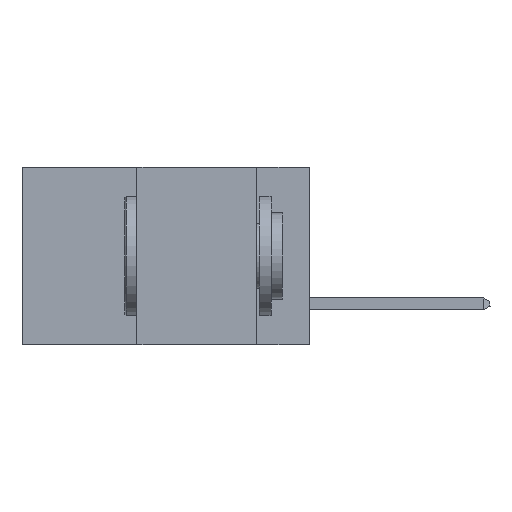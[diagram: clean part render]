
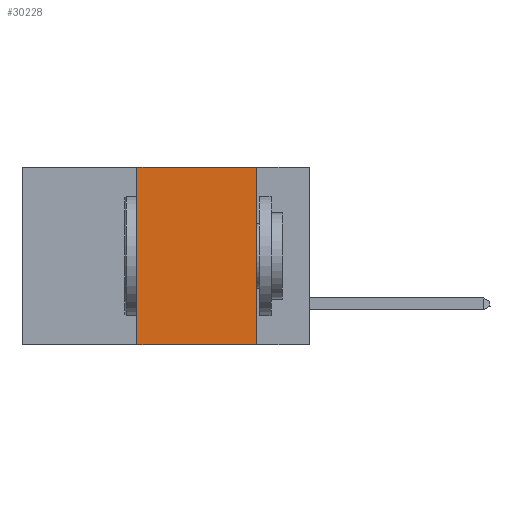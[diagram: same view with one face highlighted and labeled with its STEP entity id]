
A CAD part, left-side view. The second image highlights one B-rep face of the part: STEP entity #30228.
In plain terms, the highlighted planar face has unit normal (-1, 0, 0).
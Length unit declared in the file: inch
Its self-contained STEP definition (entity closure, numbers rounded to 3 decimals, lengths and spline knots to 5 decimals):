
#517 = VERTEX_POINT ( 'NONE', #22471 ) ;
#754 = VECTOR ( 'NONE', #20483, 39.37008 ) ;
#3112 = CARTESIAN_POINT ( 'NONE',  ( 0., 0.6, 0. ) ) ;
#3132 = CARTESIAN_POINT ( 'NONE',  ( 0., 0.11, 0. ) ) ;
#3850 = LINE ( 'NONE', #14837, #6378 ) ;
#3907 = EDGE_LOOP ( 'NONE', ( #3960, #18296, #24147, #13982 ) ) ;
#3960 = ORIENTED_EDGE ( 'NONE', *, *, #5728, .F. ) ;
#5728 = EDGE_CURVE ( 'NONE', #21485, #5902, #32385, .T. ) ;
#5902 = VERTEX_POINT ( 'NONE', #8078 ) ;
#6378 = VECTOR ( 'NONE', #7292, 39.37008 ) ;
#7025 = CARTESIAN_POINT ( 'NONE',  ( 0., 0.36, -0.37 ) ) ;
#7292 = DIRECTION ( 'NONE',  ( 0., -1., 0. ) ) ;
#8078 = CARTESIAN_POINT ( 'NONE',  ( 0., 0.11, -0.37 ) ) ;
#10292 = CARTESIAN_POINT ( 'NONE',  ( 0., 0.36, 0. ) ) ;
#11163 = DIRECTION ( 'NONE',  ( 1., 0., 0. ) ) ;
#11604 = LINE ( 'NONE', #20729, #754 ) ;
#13707 = PLANE ( 'NONE',  #33109 ) ;
#13750 = VERTEX_POINT ( 'NONE', #7025 ) ;
#13982 = ORIENTED_EDGE ( 'NONE', *, *, #25751, .T. ) ;
#14837 = CARTESIAN_POINT ( 'NONE',  ( 0., 0.6, -0.37 ) ) ;
#15100 = FACE_OUTER_BOUND ( 'NONE', #3907, .T. ) ;
#18296 = ORIENTED_EDGE ( 'NONE', *, *, #32809, .F. ) ;
#18901 = DIRECTION ( 'NONE',  ( 0., 0., -1. ) ) ;
#19064 = VECTOR ( 'NONE', #33527, 39.37008 ) ;
#19139 = CARTESIAN_POINT ( 'NONE',  ( 0., 0.11, 0. ) ) ;
#20309 = EDGE_CURVE ( 'NONE', #13750, #517, #21603, .T. ) ;
#20483 = DIRECTION ( 'NONE',  ( 0., -1., 0. ) ) ;
#20729 = CARTESIAN_POINT ( 'NONE',  ( 0., 0.6, 0. ) ) ;
#21485 = VERTEX_POINT ( 'NONE', #19139 ) ;
#21603 = LINE ( 'NONE', #10292, #19064 ) ;
#22471 = CARTESIAN_POINT ( 'NONE',  ( 0., 0.36, 0. ) ) ;
#24147 = ORIENTED_EDGE ( 'NONE', *, *, #20309, .F. ) ;
#25751 = EDGE_CURVE ( 'NONE', #13750, #5902, #3850, .T. ) ;
#27086 = DIRECTION ( 'NONE',  ( 0., 0., -1. ) ) ;
#29541 = VECTOR ( 'NONE', #18901, 39.37008 ) ;
#30228 = ADVANCED_FACE ( 'NONE', ( #15100 ), #13707, .F. ) ;
#32385 = LINE ( 'NONE', #3132, #29541 ) ;
#32809 = EDGE_CURVE ( 'NONE', #517, #21485, #11604, .T. ) ;
#33109 = AXIS2_PLACEMENT_3D ( 'NONE', #3112, #11163, #27086 ) ;
#33527 = DIRECTION ( 'NONE',  ( 0., 0., 1. ) ) ;
